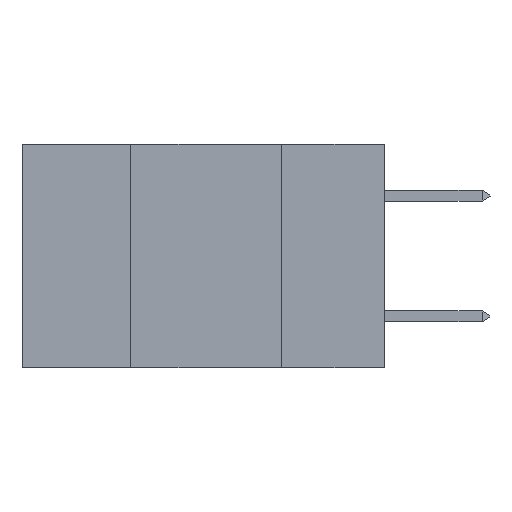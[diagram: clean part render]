
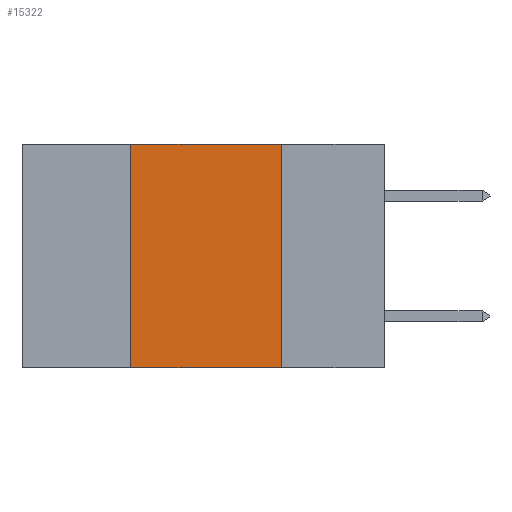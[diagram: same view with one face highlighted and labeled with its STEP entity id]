
A CAD part, left-side view. The second image highlights one B-rep face of the part: STEP entity #15322.
In plain terms, the highlighted planar face has unit normal (-1, 0, 0).
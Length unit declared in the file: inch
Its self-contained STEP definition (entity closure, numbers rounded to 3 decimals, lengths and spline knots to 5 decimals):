
#290 = EDGE_LOOP ( 'NONE', ( #29428, #295, #21667, #3582 ) ) ;
#295 = ORIENTED_EDGE ( 'NONE', *, *, #25792, .F. ) ;
#2112 = EDGE_CURVE ( 'NONE', #20524, #8927, #13094, .T. ) ;
#2679 = LINE ( 'NONE', #26103, #6957 ) ;
#3582 = ORIENTED_EDGE ( 'NONE', *, *, #4229, .T. ) ;
#4229 = EDGE_CURVE ( 'NONE', #29706, #8927, #17880, .T. ) ;
#5223 = DIRECTION ( 'NONE',  ( 0., 0., -1. ) ) ;
#5420 = DIRECTION ( 'NONE',  ( 0., 0., -1. ) ) ;
#5923 = DIRECTION ( 'NONE',  ( 0., -1., 0. ) ) ;
#6037 = DIRECTION ( 'NONE',  ( 1., 0., 0. ) ) ;
#6957 = VECTOR ( 'NONE', #9472, 39.37008 ) ;
#7151 = AXIS2_PLACEMENT_3D ( 'NONE', #24896, #6037, #5420 ) ;
#7592 = CARTESIAN_POINT ( 'NONE',  ( 0., 0.17, 0. ) ) ;
#8092 = EDGE_CURVE ( 'NONE', #29706, #27712, #18927, .T. ) ;
#8267 = PLANE ( 'NONE',  #7151 ) ;
#8927 = VERTEX_POINT ( 'NONE', #14242 ) ;
#9472 = DIRECTION ( 'NONE',  ( 0., -1., 0. ) ) ;
#10041 = CARTESIAN_POINT ( 'NONE',  ( 0., 0.42, 0. ) ) ;
#13094 = LINE ( 'NONE', #7592, #27408 ) ;
#13108 = VECTOR ( 'NONE', #5923, 39.37008 ) ;
#14242 = CARTESIAN_POINT ( 'NONE',  ( 0., 0.17, -0.37 ) ) ;
#15322 = ADVANCED_FACE ( 'NONE', ( #20190 ), #8267, .F. ) ;
#16423 = CARTESIAN_POINT ( 'NONE',  ( 0., 0.42, 0. ) ) ;
#17880 = LINE ( 'NONE', #18031, #13108 ) ;
#18031 = CARTESIAN_POINT ( 'NONE',  ( 0., 0.6, -0.37 ) ) ;
#18927 = LINE ( 'NONE', #16423, #26756 ) ;
#20190 = FACE_OUTER_BOUND ( 'NONE', #290, .T. ) ;
#20524 = VERTEX_POINT ( 'NONE', #26974 ) ;
#21667 = ORIENTED_EDGE ( 'NONE', *, *, #8092, .F. ) ;
#21749 = CARTESIAN_POINT ( 'NONE',  ( 0., 0.42, -0.37 ) ) ;
#24896 = CARTESIAN_POINT ( 'NONE',  ( 0., 0.6, 0. ) ) ;
#25792 = EDGE_CURVE ( 'NONE', #27712, #20524, #2679, .T. ) ;
#26103 = CARTESIAN_POINT ( 'NONE',  ( 0., 0.6, 0. ) ) ;
#26756 = VECTOR ( 'NONE', #28039, 39.37008 ) ;
#26974 = CARTESIAN_POINT ( 'NONE',  ( 0., 0.17, 0. ) ) ;
#27408 = VECTOR ( 'NONE', #5223, 39.37008 ) ;
#27712 = VERTEX_POINT ( 'NONE', #10041 ) ;
#28039 = DIRECTION ( 'NONE',  ( 0., 0., 1. ) ) ;
#29428 = ORIENTED_EDGE ( 'NONE', *, *, #2112, .F. ) ;
#29706 = VERTEX_POINT ( 'NONE', #21749 ) ;
